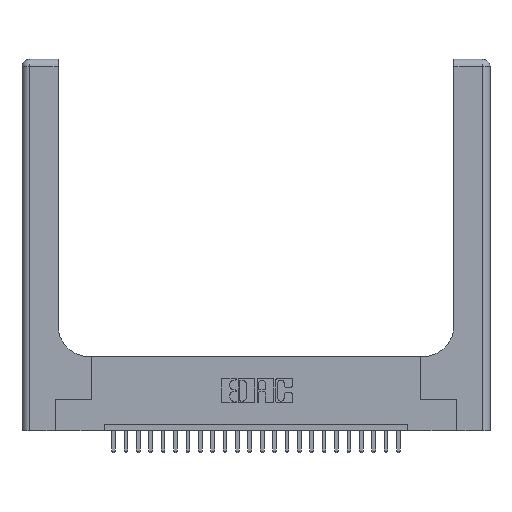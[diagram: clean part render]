
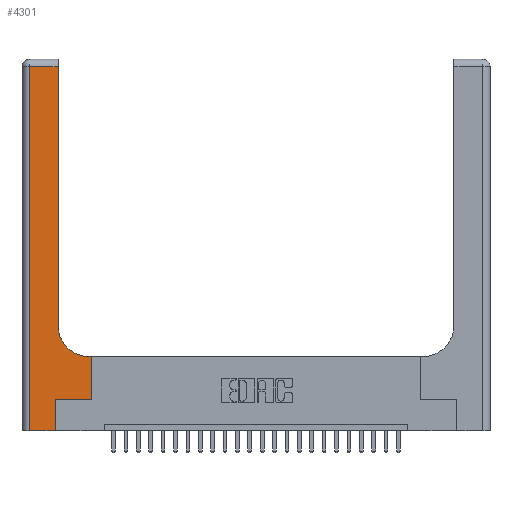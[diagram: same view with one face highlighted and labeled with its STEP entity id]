
A CAD part, top view. The second image highlights one B-rep face of the part: STEP entity #4301.
In plain terms, the highlighted planar face has unit normal (0, 0, 1).
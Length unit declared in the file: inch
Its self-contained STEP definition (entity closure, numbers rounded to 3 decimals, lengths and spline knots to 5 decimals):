
#597 = VECTOR ( 'NONE', #11830, 39.37008 ) ;
#771 = DIRECTION ( 'NONE',  ( -1., 0., 0. ) ) ;
#1073 = DIRECTION ( 'NONE',  ( 0., 1., 0. ) ) ;
#1917 = VECTOR ( 'NONE', #1073, 39.37008 ) ;
#2082 = EDGE_CURVE ( 'NONE', #14277, #8492, #22850, .T. ) ;
#2136 = CARTESIAN_POINT ( 'NONE',  ( 0.269, 0.25, 0.37 ) ) ;
#2322 = EDGE_CURVE ( 'NONE', #2511, #14277, #17254, .T. ) ;
#2323 = LINE ( 'NONE', #3800, #5739 ) ;
#2511 = VERTEX_POINT ( 'NONE', #15347 ) ;
#3161 = FACE_OUTER_BOUND ( 'NONE', #7342, .T. ) ;
#3800 = CARTESIAN_POINT ( 'NONE',  ( 0.06, 3., 0.37 ) ) ;
#4301 = ADVANCED_FACE ( 'NONE', ( #3161 ), #18257, .F. ) ;
#5739 = VECTOR ( 'NONE', #9756, 39.37008 ) ;
#5867 = VECTOR ( 'NONE', #10512, 39.37008 ) ;
#6690 = DIRECTION ( 'NONE',  ( 0., 0., -1. ) ) ;
#6968 = EDGE_CURVE ( 'NONE', #13342, #21384, #8357, .T. ) ;
#7018 = CARTESIAN_POINT ( 'NONE',  ( 0., 3., 0.37 ) ) ;
#7342 = EDGE_LOOP ( 'NONE', ( #15176, #20521, #23145, #23926, #8731, #24078, #16020, #24757, #22165 ) ) ;
#7446 = CARTESIAN_POINT ( 'NONE',  ( 0.5585, 0.25, 0.37 ) ) ;
#8091 = EDGE_CURVE ( 'NONE', #14299, #18089, #10208, .T. ) ;
#8325 = CARTESIAN_POINT ( 'NONE',  ( 0.2915, 0.6, 0.37 ) ) ;
#8357 = LINE ( 'NONE', #8325, #5867 ) ;
#8492 = VERTEX_POINT ( 'NONE', #7446 ) ;
#8666 = EDGE_CURVE ( 'NONE', #18089, #21152, #15183, .T. ) ;
#8698 = AXIS2_PLACEMENT_3D ( 'NONE', #21376, #19353, #25329 ) ;
#8731 = ORIENTED_EDGE ( 'NONE', *, *, #2322, .T. ) ;
#8898 = DIRECTION ( 'NONE',  ( -1., 0., 0. ) ) ;
#9092 = AXIS2_PLACEMENT_3D ( 'NONE', #7018, #6690, #771 ) ;
#9756 = DIRECTION ( 'NONE',  ( 0., -1., 0. ) ) ;
#9873 = VECTOR ( 'NONE', #8898, 39.37008 ) ;
#9882 = CARTESIAN_POINT ( 'NONE',  ( 0.2915, 2.94, 0.37 ) ) ;
#10208 = LINE ( 'NONE', #20891, #13630 ) ;
#10512 = DIRECTION ( 'NONE',  ( -1., 0., 0. ) ) ;
#11662 = DIRECTION ( 'NONE',  ( 1., 0., 0. ) ) ;
#11830 = DIRECTION ( 'NONE',  ( 1., 0., 0. ) ) ;
#11838 = CARTESIAN_POINT ( 'NONE',  ( 0.269, 0.25, 0.37 ) ) ;
#12936 = EDGE_CURVE ( 'NONE', #21152, #21217, #2323, .T. ) ;
#13049 = CARTESIAN_POINT ( 'NONE',  ( 0.269, 0., 0.37 ) ) ;
#13342 = VERTEX_POINT ( 'NONE', #21089 ) ;
#13630 = VECTOR ( 'NONE', #24446, 39.37008 ) ;
#14277 = VERTEX_POINT ( 'NONE', #2136 ) ;
#14299 = VERTEX_POINT ( 'NONE', #20250 ) ;
#14451 = EDGE_CURVE ( 'NONE', #8492, #13342, #19701, .T. ) ;
#15176 = ORIENTED_EDGE ( 'NONE', *, *, #8091, .T. ) ;
#15183 = LINE ( 'NONE', #24425, #9873 ) ;
#15347 = CARTESIAN_POINT ( 'NONE',  ( 0.269, 0., 0.37 ) ) ;
#15765 = CARTESIAN_POINT ( 'NONE',  ( 0., 0., 0.37 ) ) ;
#16020 = ORIENTED_EDGE ( 'NONE', *, *, #14451, .T. ) ;
#16725 = CARTESIAN_POINT ( 'NONE',  ( 0.5585, 0.25, 0.37 ) ) ;
#17254 = LINE ( 'NONE', #13049, #21322 ) ;
#17890 = CIRCLE ( 'NONE', #8698, 0.25 ) ;
#18089 = VERTEX_POINT ( 'NONE', #9882 ) ;
#18257 = PLANE ( 'NONE',  #9092 ) ;
#19232 = EDGE_CURVE ( 'NONE', #21217, #2511, #22076, .T. ) ;
#19353 = DIRECTION ( 'NONE',  ( 0., 0., -1. ) ) ;
#19701 = LINE ( 'NONE', #16725, #1917 ) ;
#20250 = CARTESIAN_POINT ( 'NONE',  ( 0.2915, 0.85, 0.37 ) ) ;
#20521 = ORIENTED_EDGE ( 'NONE', *, *, #8666, .T. ) ;
#20891 = CARTESIAN_POINT ( 'NONE',  ( 0.2915, 3., 0.37 ) ) ;
#20943 = DIRECTION ( 'NONE',  ( 0., 1., 0. ) ) ;
#21089 = CARTESIAN_POINT ( 'NONE',  ( 0.5585, 0.6, 0.37 ) ) ;
#21152 = VERTEX_POINT ( 'NONE', #22861 ) ;
#21217 = VERTEX_POINT ( 'NONE', #21335 ) ;
#21322 = VECTOR ( 'NONE', #20943, 39.37008 ) ;
#21335 = CARTESIAN_POINT ( 'NONE',  ( 0.06, 0., 0.37 ) ) ;
#21376 = CARTESIAN_POINT ( 'NONE',  ( 0.5415, 0.85, 0.37 ) ) ;
#21384 = VERTEX_POINT ( 'NONE', #25782 ) ;
#22076 = LINE ( 'NONE', #15765, #597 ) ;
#22165 = ORIENTED_EDGE ( 'NONE', *, *, #22928, .T. ) ;
#22208 = VECTOR ( 'NONE', #11662, 39.37008 ) ;
#22850 = LINE ( 'NONE', #11838, #22208 ) ;
#22861 = CARTESIAN_POINT ( 'NONE',  ( 0.06, 2.94, 0.37 ) ) ;
#22928 = EDGE_CURVE ( 'NONE', #21384, #14299, #17890, .T. ) ;
#23145 = ORIENTED_EDGE ( 'NONE', *, *, #12936, .T. ) ;
#23926 = ORIENTED_EDGE ( 'NONE', *, *, #19232, .T. ) ;
#24078 = ORIENTED_EDGE ( 'NONE', *, *, #2082, .T. ) ;
#24425 = CARTESIAN_POINT ( 'NONE',  ( 0., 2.94, 0.37 ) ) ;
#24446 = DIRECTION ( 'NONE',  ( 0., 1., 0. ) ) ;
#24757 = ORIENTED_EDGE ( 'NONE', *, *, #6968, .T. ) ;
#25329 = DIRECTION ( 'NONE',  ( 1., 0., 0. ) ) ;
#25782 = CARTESIAN_POINT ( 'NONE',  ( 0.5415, 0.6, 0.37 ) ) ;
